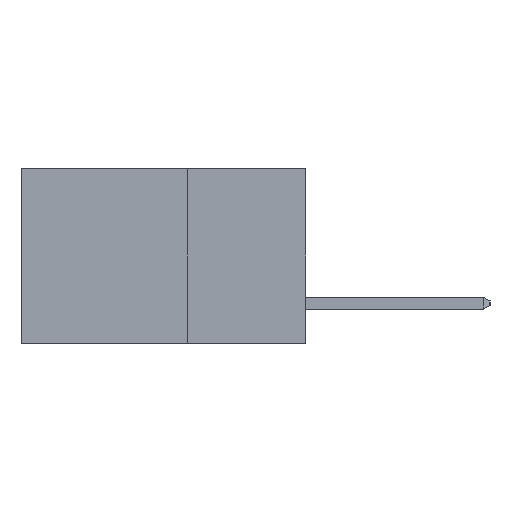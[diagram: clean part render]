
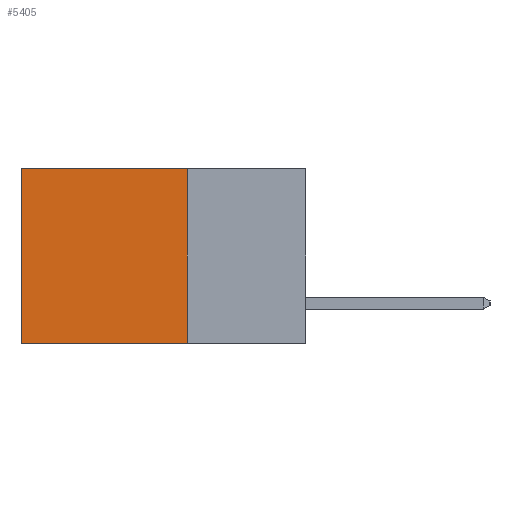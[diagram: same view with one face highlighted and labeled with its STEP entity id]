
A CAD part, left-side view. The second image highlights one B-rep face of the part: STEP entity #5405.
In plain terms, the highlighted planar face has unit normal (-1, 0, 0).
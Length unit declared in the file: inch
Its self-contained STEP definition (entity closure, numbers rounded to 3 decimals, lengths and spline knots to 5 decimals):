
#738 = CARTESIAN_POINT ( 'NONE',  ( 0.298, 0.6, 0. ) ) ;
#915 = VERTEX_POINT ( 'NONE', #20216 ) ;
#1360 = EDGE_CURVE ( 'NONE', #21155, #915, #8496, .T. ) ;
#4467 = DIRECTION ( 'NONE',  ( 0., 1., 0. ) ) ;
#4569 = EDGE_CURVE ( 'NONE', #13590, #12457, #21131, .T. ) ;
#5405 = ADVANCED_FACE ( 'NONE', ( #8538 ), #15705, .F. ) ;
#6446 = ORIENTED_EDGE ( 'NONE', *, *, #1360, .T. ) ;
#6832 = ORIENTED_EDGE ( 'NONE', *, *, #7945, .T. ) ;
#7558 = EDGE_LOOP ( 'NONE', ( #6446, #13543, #7678, #6832 ) ) ;
#7678 = ORIENTED_EDGE ( 'NONE', *, *, #4569, .F. ) ;
#7945 = EDGE_CURVE ( 'NONE', #13590, #21155, #20423, .T. ) ;
#8046 = VECTOR ( 'NONE', #19451, 39.37008 ) ;
#8496 = LINE ( 'NONE', #14322, #20561 ) ;
#8538 = FACE_OUTER_BOUND ( 'NONE', #7558, .T. ) ;
#10173 = CARTESIAN_POINT ( 'NONE',  ( 0.298, 0.25, 0. ) ) ;
#12457 = VERTEX_POINT ( 'NONE', #17586 ) ;
#12553 = VECTOR ( 'NONE', #4467, 39.37008 ) ;
#13000 = CARTESIAN_POINT ( 'NONE',  ( 0.298, 0.25, 0. ) ) ;
#13543 = ORIENTED_EDGE ( 'NONE', *, *, #18834, .F. ) ;
#13590 = VERTEX_POINT ( 'NONE', #13000 ) ;
#14322 = CARTESIAN_POINT ( 'NONE',  ( 0.298, 0.6, 0. ) ) ;
#14659 = DIRECTION ( 'NONE',  ( 0., 0., -1. ) ) ;
#15705 = PLANE ( 'NONE',  #17273 ) ;
#16081 = CARTESIAN_POINT ( 'NONE',  ( 0.298, 0.25, -0.37 ) ) ;
#16708 = DIRECTION ( 'NONE',  ( 1., 0., 0. ) ) ;
#16876 = CARTESIAN_POINT ( 'NONE',  ( 0.298, 0.25, 0. ) ) ;
#16897 = DIRECTION ( 'NONE',  ( 0., 1., 0. ) ) ;
#16908 = LINE ( 'NONE', #16081, #12553 ) ;
#17273 = AXIS2_PLACEMENT_3D ( 'NONE', #10173, #16708, #18223 ) ;
#17447 = CARTESIAN_POINT ( 'NONE',  ( 0.298, 0.25, 0. ) ) ;
#17586 = CARTESIAN_POINT ( 'NONE',  ( 0.298, 0.25, -0.37 ) ) ;
#18223 = DIRECTION ( 'NONE',  ( 0., 0., -1. ) ) ;
#18834 = EDGE_CURVE ( 'NONE', #12457, #915, #16908, .T. ) ;
#19451 = DIRECTION ( 'NONE',  ( 0., 0., -1. ) ) ;
#19907 = VECTOR ( 'NONE', #16897, 39.37008 ) ;
#20216 = CARTESIAN_POINT ( 'NONE',  ( 0.298, 0.6, -0.37 ) ) ;
#20423 = LINE ( 'NONE', #16876, #19907 ) ;
#20561 = VECTOR ( 'NONE', #14659, 39.37008 ) ;
#21131 = LINE ( 'NONE', #17447, #8046 ) ;
#21155 = VERTEX_POINT ( 'NONE', #738 ) ;
